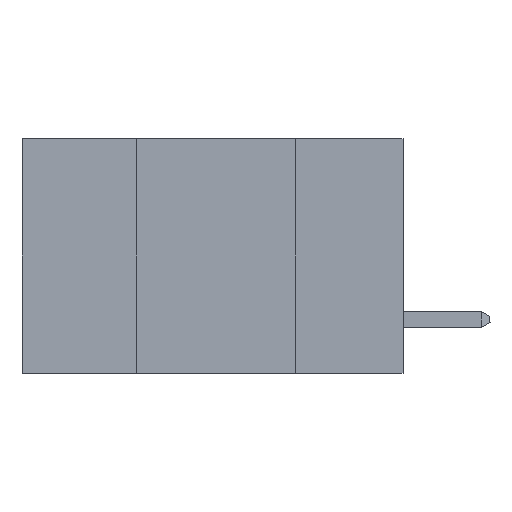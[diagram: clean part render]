
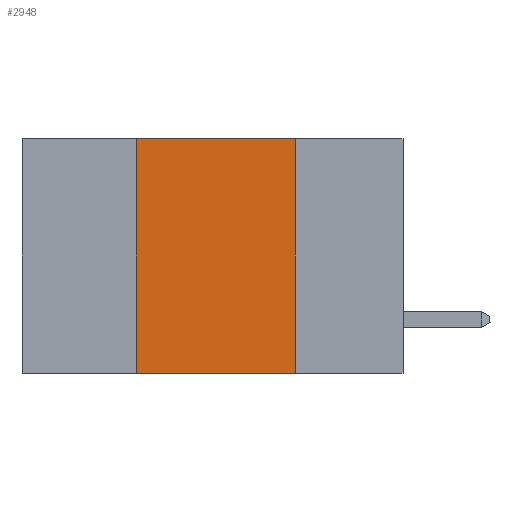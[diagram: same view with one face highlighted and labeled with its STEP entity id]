
A CAD part, left-side view. The second image highlights one B-rep face of the part: STEP entity #2948.
In plain terms, the highlighted planar face has unit normal (-1, 0, 0).
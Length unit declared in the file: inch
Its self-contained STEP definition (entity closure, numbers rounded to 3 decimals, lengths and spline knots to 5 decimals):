
#180 = VECTOR ( 'NONE', #18059, 39.37008 ) ;
#577 = CARTESIAN_POINT ( 'NONE',  ( 0., 0.6, 0. ) ) ;
#2948 = ADVANCED_FACE ( 'NONE', ( #14215 ), #30674, .F. ) ;
#3337 = ORIENTED_EDGE ( 'NONE', *, *, #25411, .F. ) ;
#4136 = DIRECTION ( 'NONE',  ( 0., -1., 0. ) ) ;
#4707 = VECTOR ( 'NONE', #4136, 39.37008 ) ;
#5416 = EDGE_CURVE ( 'NONE', #29718, #30496, #13925, .T. ) ;
#6258 = LINE ( 'NONE', #11476, #27306 ) ;
#6610 = CARTESIAN_POINT ( 'NONE',  ( 0., 0.6, -0.37 ) ) ;
#7413 = VERTEX_POINT ( 'NONE', #30776 ) ;
#7616 = ORIENTED_EDGE ( 'NONE', *, *, #5416, .T. ) ;
#8286 = VERTEX_POINT ( 'NONE', #35040 ) ;
#11476 = CARTESIAN_POINT ( 'NONE',  ( 0., 0.17, 0. ) ) ;
#12069 = DIRECTION ( 'NONE',  ( 1., 0., 0. ) ) ;
#12262 = DIRECTION ( 'NONE',  ( 0., 0., 1. ) ) ;
#13680 = CARTESIAN_POINT ( 'NONE',  ( 0., 0.42, -0.37 ) ) ;
#13925 = LINE ( 'NONE', #6610, #180 ) ;
#14215 = FACE_OUTER_BOUND ( 'NONE', #23927, .T. ) ;
#18059 = DIRECTION ( 'NONE',  ( 0., -1., 0. ) ) ;
#19375 = LINE ( 'NONE', #23435, #4707 ) ;
#21153 = LINE ( 'NONE', #23202, #27484 ) ;
#23202 = CARTESIAN_POINT ( 'NONE',  ( 0., 0.42, 0. ) ) ;
#23435 = CARTESIAN_POINT ( 'NONE',  ( 0., 0.6, 0. ) ) ;
#23927 = EDGE_LOOP ( 'NONE', ( #25294, #27013, #3337, #7616 ) ) ;
#25294 = ORIENTED_EDGE ( 'NONE', *, *, #32013, .F. ) ;
#25411 = EDGE_CURVE ( 'NONE', #29718, #7413, #21153, .T. ) ;
#25458 = EDGE_CURVE ( 'NONE', #7413, #8286, #19375, .T. ) ;
#27013 = ORIENTED_EDGE ( 'NONE', *, *, #25458, .F. ) ;
#27306 = VECTOR ( 'NONE', #30592, 39.37008 ) ;
#27484 = VECTOR ( 'NONE', #12262, 39.37008 ) ;
#29642 = CARTESIAN_POINT ( 'NONE',  ( 0., 0.17, -0.37 ) ) ;
#29718 = VERTEX_POINT ( 'NONE', #13680 ) ;
#30496 = VERTEX_POINT ( 'NONE', #29642 ) ;
#30592 = DIRECTION ( 'NONE',  ( 0., 0., -1. ) ) ;
#30674 = PLANE ( 'NONE',  #33136 ) ;
#30776 = CARTESIAN_POINT ( 'NONE',  ( 0., 0.42, 0. ) ) ;
#32013 = EDGE_CURVE ( 'NONE', #8286, #30496, #6258, .T. ) ;
#33136 = AXIS2_PLACEMENT_3D ( 'NONE', #577, #12069, #35313 ) ;
#35040 = CARTESIAN_POINT ( 'NONE',  ( 0., 0.17, 0. ) ) ;
#35313 = DIRECTION ( 'NONE',  ( 0., 0., -1. ) ) ;
